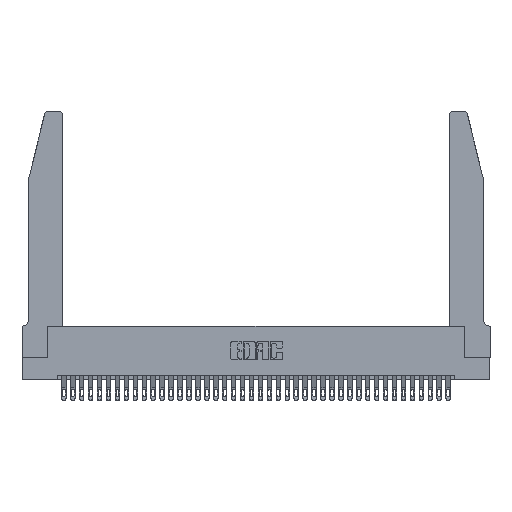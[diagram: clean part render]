
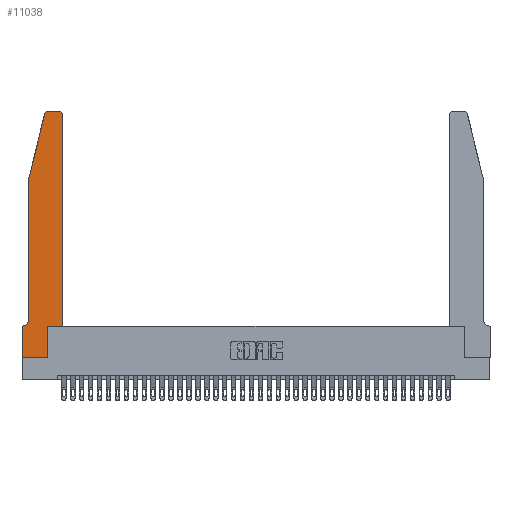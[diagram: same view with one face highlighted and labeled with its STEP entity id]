
A CAD part, top view. The second image highlights one B-rep face of the part: STEP entity #11038.
In plain terms, the highlighted planar face has unit normal (0, 0, 1).
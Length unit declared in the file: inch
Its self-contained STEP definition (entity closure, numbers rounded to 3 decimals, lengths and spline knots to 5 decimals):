
#1732 = DIRECTION ( 'NONE',  ( -1., 0., 0. ) ) ;
#2064 = LINE ( 'NONE', #25653, #29592 ) ;
#2380 = EDGE_CURVE ( 'NONE', #8024, #33606, #23602, .T. ) ;
#3351 = AXIS2_PLACEMENT_3D ( 'NONE', #14146, #14399, #17187 ) ;
#3458 = DIRECTION ( 'NONE',  ( 1., 0., 0. ) ) ;
#4231 = PLANE ( 'NONE',  #23656 ) ;
#4528 = VECTOR ( 'NONE', #13370, 39.37008 ) ;
#5011 = ORIENTED_EDGE ( 'NONE', *, *, #8276, .T. ) ;
#5196 = VECTOR ( 'NONE', #3458, 39.37008 ) ;
#5529 = CARTESIAN_POINT ( 'NONE',  ( 0.0055, 0.42, 0.37 ) ) ;
#5855 = VERTEX_POINT ( 'NONE', #30127 ) ;
#6375 = ORIENTED_EDGE ( 'NONE', *, *, #8966, .T. ) ;
#7286 = ORIENTED_EDGE ( 'NONE', *, *, #24528, .T. ) ;
#7293 = CARTESIAN_POINT ( 'NONE',  ( 0.2865, 0.35, 0.37 ) ) ;
#8024 = VERTEX_POINT ( 'NONE', #36220 ) ;
#8276 = EDGE_CURVE ( 'NONE', #33606, #15642, #20325, .T. ) ;
#8329 = DIRECTION ( 'NONE',  ( 1., 0., 0. ) ) ;
#8394 = VERTEX_POINT ( 'NONE', #19931 ) ;
#8566 = DIRECTION ( 'NONE',  ( 0., 0., -1. ) ) ;
#8602 = CARTESIAN_POINT ( 'NONE',  ( 0.0755, 0.42, 0.37 ) ) ;
#8966 = EDGE_CURVE ( 'NONE', #22630, #36933, #14562, .T. ) ;
#9278 = AXIS2_PLACEMENT_3D ( 'NONE', #37261, #12674, #30748 ) ;
#9357 = EDGE_CURVE ( 'NONE', #9596, #21886, #30700, .T. ) ;
#9596 = VERTEX_POINT ( 'NONE', #19016 ) ;
#9912 = DIRECTION ( 'NONE',  ( -0.239, -0.971, 0. ) ) ;
#9955 = ORIENTED_EDGE ( 'NONE', *, *, #32820, .T. ) ;
#10642 = CARTESIAN_POINT ( 'NONE',  ( 0.4505, 0.35, 0.37 ) ) ;
#10858 = CARTESIAN_POINT ( 'NONE',  ( 0., 0.35, 0.37 ) ) ;
#11038 = ADVANCED_FACE ( 'NONE', ( #27261 ), #4231, .T. ) ;
#11248 = ORIENTED_EDGE ( 'NONE', *, *, #14744, .T. ) ;
#12069 = VECTOR ( 'NONE', #8329, 39.37008 ) ;
#12668 = CARTESIAN_POINT ( 'NONE',  ( 0.0755, 0.35, 0.37 ) ) ;
#12674 = DIRECTION ( 'NONE',  ( 0., 0., 1. ) ) ;
#13370 = DIRECTION ( 'NONE',  ( 0., 1., 0. ) ) ;
#13863 = VECTOR ( 'NONE', #1732, 39.37008 ) ;
#14070 = CIRCLE ( 'NONE', #9278, 0.03 ) ;
#14146 = CARTESIAN_POINT ( 'NONE',  ( 0.284, 2.72, 0.37 ) ) ;
#14399 = DIRECTION ( 'NONE',  ( 0., 0., 1. ) ) ;
#14562 = CIRCLE ( 'NONE', #22843, 0.07 ) ;
#14630 = DIRECTION ( 'NONE',  ( -1., 0., 0. ) ) ;
#14717 = EDGE_LOOP ( 'NONE', ( #37921, #18270, #5011, #36186, #6375, #9955, #36569, #31701, #7286, #35949, #21480, #11248 ) ) ;
#14744 = EDGE_CURVE ( 'NONE', #8394, #31342, #14070, .T. ) ;
#15642 = VERTEX_POINT ( 'NONE', #34516 ) ;
#15736 = LINE ( 'NONE', #38129, #13863 ) ;
#16143 = VECTOR ( 'NONE', #18489, 39.37008 ) ;
#16354 = LINE ( 'NONE', #7293, #4528 ) ;
#16995 = EDGE_CURVE ( 'NONE', #35180, #8394, #2064, .T. ) ;
#17187 = DIRECTION ( 'NONE',  ( 1., 0., 0. ) ) ;
#17198 = DIRECTION ( 'NONE',  ( 0., 0., 1. ) ) ;
#18270 = ORIENTED_EDGE ( 'NONE', *, *, #2380, .T. ) ;
#18489 = DIRECTION ( 'NONE',  ( -1., 0., 0. ) ) ;
#18557 = LINE ( 'NONE', #38323, #35725 ) ;
#18824 = CARTESIAN_POINT ( 'NONE',  ( 0.25487, 2.72718, 0.37 ) ) ;
#19016 = CARTESIAN_POINT ( 'NONE',  ( 0., 0.35, 0.37 ) ) ;
#19931 = CARTESIAN_POINT ( 'NONE',  ( 0.4505, 2.72, 0.37 ) ) ;
#20099 = DIRECTION ( 'NONE',  ( 0., -1., 0. ) ) ;
#20123 = EDGE_CURVE ( 'NONE', #15642, #22630, #18557, .T. ) ;
#20263 = DIRECTION ( 'NONE',  ( 0., -1., 0. ) ) ;
#20325 = LINE ( 'NONE', #25040, #22681 ) ;
#21480 = ORIENTED_EDGE ( 'NONE', *, *, #16995, .T. ) ;
#21637 = EDGE_CURVE ( 'NONE', #25864, #35180, #38922, .T. ) ;
#21886 = VERTEX_POINT ( 'NONE', #28899 ) ;
#22630 = VERTEX_POINT ( 'NONE', #8602 ) ;
#22681 = VECTOR ( 'NONE', #9912, 39.37008 ) ;
#22843 = AXIS2_PLACEMENT_3D ( 'NONE', #5529, #8566, #14630 ) ;
#23602 = CIRCLE ( 'NONE', #3351, 0.03 ) ;
#23656 = AXIS2_PLACEMENT_3D ( 'NONE', #10858, #17198, #35437 ) ;
#24528 = EDGE_CURVE ( 'NONE', #5855, #25864, #16354, .T. ) ;
#25040 = CARTESIAN_POINT ( 'NONE',  ( 0.0755, 2., 0.37 ) ) ;
#25653 = CARTESIAN_POINT ( 'NONE',  ( 0.4505, 0.35, 0.37 ) ) ;
#25864 = VERTEX_POINT ( 'NONE', #32146 ) ;
#26864 = CARTESIAN_POINT ( 'NONE',  ( 0.4205, 2.75, 0.37 ) ) ;
#27261 = FACE_OUTER_BOUND ( 'NONE', #14717, .T. ) ;
#28535 = LINE ( 'NONE', #12668, #16143 ) ;
#28704 = DIRECTION ( 'NONE',  ( 0., 1., 0. ) ) ;
#28899 = CARTESIAN_POINT ( 'NONE',  ( 0., 0., 0.37 ) ) ;
#29257 = EDGE_CURVE ( 'NONE', #21886, #5855, #30128, .T. ) ;
#29592 = VECTOR ( 'NONE', #28704, 39.37008 ) ;
#30127 = CARTESIAN_POINT ( 'NONE',  ( 0.2865, 0., 0.37 ) ) ;
#30128 = LINE ( 'NONE', #38448, #12069 ) ;
#30527 = CARTESIAN_POINT ( 'NONE',  ( 0.4505, 0.35, 0.37 ) ) ;
#30700 = LINE ( 'NONE', #35431, #31141 ) ;
#30748 = DIRECTION ( 'NONE',  ( 1., 0., 0. ) ) ;
#31141 = VECTOR ( 'NONE', #20263, 39.37008 ) ;
#31342 = VERTEX_POINT ( 'NONE', #26864 ) ;
#31701 = ORIENTED_EDGE ( 'NONE', *, *, #29257, .T. ) ;
#31818 = EDGE_CURVE ( 'NONE', #31342, #8024, #15736, .T. ) ;
#32146 = CARTESIAN_POINT ( 'NONE',  ( 0.2865, 0.35, 0.37 ) ) ;
#32241 = CARTESIAN_POINT ( 'NONE',  ( 0.0055, 0.35, 0.37 ) ) ;
#32820 = EDGE_CURVE ( 'NONE', #36933, #9596, #28535, .T. ) ;
#33606 = VERTEX_POINT ( 'NONE', #18824 ) ;
#34516 = CARTESIAN_POINT ( 'NONE',  ( 0.0755, 2., 0.37 ) ) ;
#35180 = VERTEX_POINT ( 'NONE', #10642 ) ;
#35431 = CARTESIAN_POINT ( 'NONE',  ( 0., 0., 0.37 ) ) ;
#35437 = DIRECTION ( 'NONE',  ( 1., 0., 0. ) ) ;
#35725 = VECTOR ( 'NONE', #20099, 39.37008 ) ;
#35949 = ORIENTED_EDGE ( 'NONE', *, *, #21637, .T. ) ;
#36186 = ORIENTED_EDGE ( 'NONE', *, *, #20123, .T. ) ;
#36220 = CARTESIAN_POINT ( 'NONE',  ( 0.284, 2.75, 0.37 ) ) ;
#36569 = ORIENTED_EDGE ( 'NONE', *, *, #9357, .T. ) ;
#36933 = VERTEX_POINT ( 'NONE', #32241 ) ;
#37261 = CARTESIAN_POINT ( 'NONE',  ( 0.4205, 2.72, 0.37 ) ) ;
#37921 = ORIENTED_EDGE ( 'NONE', *, *, #31818, .T. ) ;
#38129 = CARTESIAN_POINT ( 'NONE',  ( 0.2605, 2.75, 0.37 ) ) ;
#38323 = CARTESIAN_POINT ( 'NONE',  ( 0.0755, 2., 0.37 ) ) ;
#38448 = CARTESIAN_POINT ( 'NONE',  ( 0., 0., 0.37 ) ) ;
#38922 = LINE ( 'NONE', #30527, #5196 ) ;
